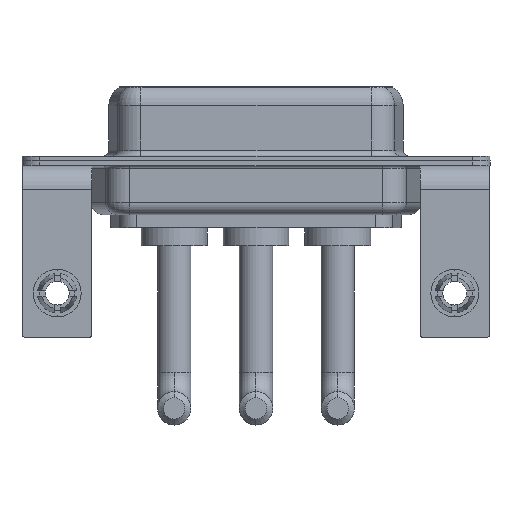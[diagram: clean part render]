
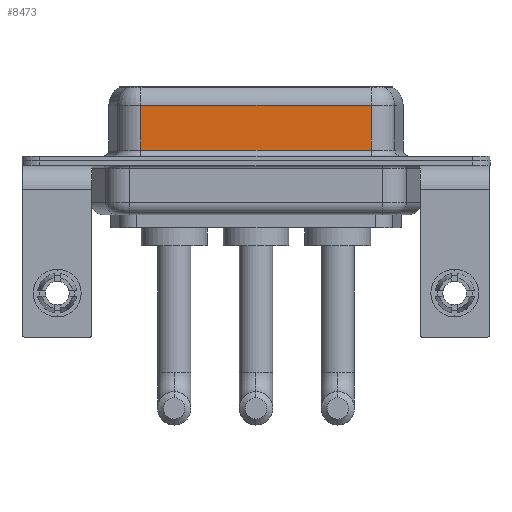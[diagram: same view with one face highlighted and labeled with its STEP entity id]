
A CAD part, front view. The second image highlights one B-rep face of the part: STEP entity #8473.
In plain terms, the highlighted planar face has unit normal (0, -1, 0).
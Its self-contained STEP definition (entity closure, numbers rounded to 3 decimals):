
#98 = DIRECTION ( 'NONE',  ( 0., 0., 1. ) ) ;
#442 = VERTEX_POINT ( 'NONE', #5591 ) ;
#1211 = FACE_OUTER_BOUND ( 'NONE', #7858, .T. ) ;
#1624 = LINE ( 'NONE', #7218, #10504 ) ;
#1796 = DIRECTION ( 'NONE',  ( -1., 0., 0. ) ) ;
#2497 = CARTESIAN_POINT ( 'NONE',  ( 26.287, -3.95, 6.4 ) ) ;
#3027 = CARTESIAN_POINT ( 'NONE',  ( 7.013, -3.95, 0.9 ) ) ;
#3107 = CARTESIAN_POINT ( 'NONE',  ( 26.287, -3.95, 0.9 ) ) ;
#3479 = CARTESIAN_POINT ( 'NONE',  ( 7.013, -3.95, 4.65 ) ) ;
#4089 = VECTOR ( 'NONE', #1796, 1000. ) ;
#5057 = CARTESIAN_POINT ( 'NONE',  ( 26.287, -3.95, 4.65 ) ) ;
#5173 = EDGE_CURVE ( 'NONE', #11719, #11594, #1624, .T. ) ;
#5339 = LINE ( 'NONE', #3107, #12647 ) ;
#5475 = EDGE_CURVE ( 'NONE', #11594, #442, #5339, .T. ) ;
#5499 = ORIENTED_EDGE ( 'NONE', *, *, #5173, .T. ) ;
#5591 = CARTESIAN_POINT ( 'NONE',  ( 26.287, -3.95, 0.9 ) ) ;
#5741 = PLANE ( 'NONE',  #13892 ) ;
#6249 = EDGE_CURVE ( 'NONE', #6771, #11719, #7606, .T. ) ;
#6771 = VERTEX_POINT ( 'NONE', #13411 ) ;
#6942 = DIRECTION ( 'NONE',  ( 0., 1., 0. ) ) ;
#7040 = DIRECTION ( 'NONE',  ( 0., 0., -1. ) ) ;
#7218 = CARTESIAN_POINT ( 'NONE',  ( 7.013, -3.95, 6.4 ) ) ;
#7606 = LINE ( 'NONE', #5057, #4089 ) ;
#7660 = DIRECTION ( 'NONE',  ( 1., 0., 0. ) ) ;
#7858 = EDGE_LOOP ( 'NONE', ( #8567, #9256, #5499, #14353 ) ) ;
#8473 = ADVANCED_FACE ( 'NONE', ( #1211 ), #5741, .F. ) ;
#8567 = ORIENTED_EDGE ( 'NONE', *, *, #14176, .F. ) ;
#9256 = ORIENTED_EDGE ( 'NONE', *, *, #6249, .T. ) ;
#10294 = CARTESIAN_POINT ( 'NONE',  ( 26.287, -3.95, 6.4 ) ) ;
#10504 = VECTOR ( 'NONE', #14155, 1000. ) ;
#10883 = VECTOR ( 'NONE', #7040, 1000. ) ;
#11594 = VERTEX_POINT ( 'NONE', #3027 ) ;
#11719 = VERTEX_POINT ( 'NONE', #3479 ) ;
#12647 = VECTOR ( 'NONE', #7660, 1000. ) ;
#12707 = LINE ( 'NONE', #2497, #10883 ) ;
#13411 = CARTESIAN_POINT ( 'NONE',  ( 26.287, -3.95, 4.65 ) ) ;
#13892 = AXIS2_PLACEMENT_3D ( 'NONE', #10294, #6942, #98 ) ;
#14155 = DIRECTION ( 'NONE',  ( 0., 0., -1. ) ) ;
#14176 = EDGE_CURVE ( 'NONE', #6771, #442, #12707, .T. ) ;
#14353 = ORIENTED_EDGE ( 'NONE', *, *, #5475, .T. ) ;
